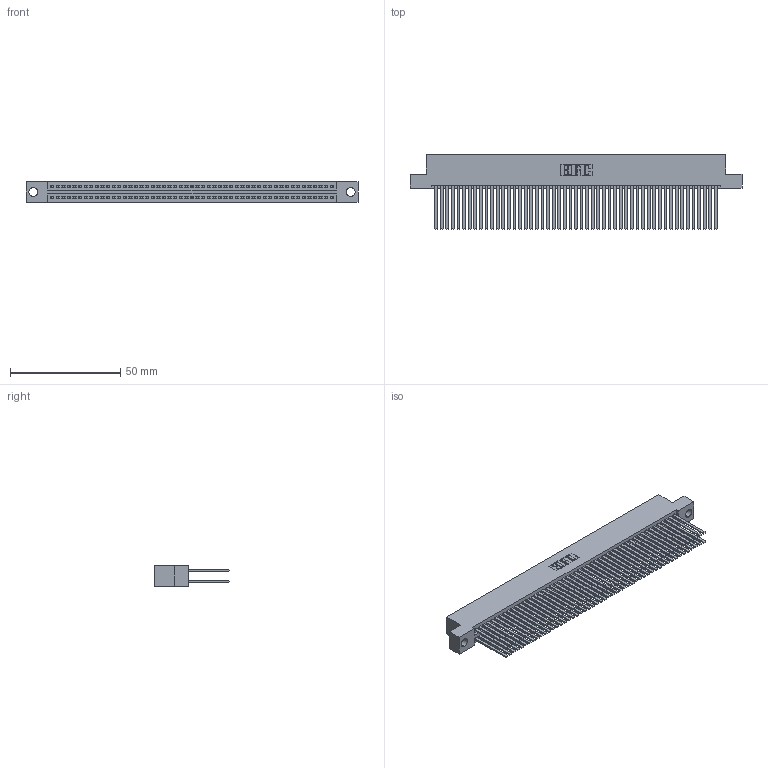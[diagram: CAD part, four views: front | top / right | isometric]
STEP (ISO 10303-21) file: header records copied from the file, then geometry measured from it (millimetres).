
FILE_DESCRIPTION (( 'STEP AP203' ), '1' );
FILE_NAME ('395-102-544-204.STEP', '2018-11-30T08:10:11', ( '' ), ( '' ), 'SwSTEP 2.0', 'SolidWorks 2016', '' );
FILE_SCHEMA (( 'CONFIG_CONTROL_DESIGN' ));
Length unit declared in the file: inch
Products named in the file (3): 345-292-001_345-293-144; 395-102-544-204; 345 Part_Flush Mounting Lugs - 0.156 Dia-TH
Assembly tree (103 placements, depth 2):
  395-102-544-204
    345 Part_Flush Mounting Lugs - 0.156 Dia-TH
    345-292-001_345-293-144  x102
Bounding box: 150.75 x 33.96 x 9.4 mm (x, y, z)
Volume: 16069.4 mm3; surface area: 27933.6 mm2
Topology: 103 solids, 103 shells, 4614 faces, 13703 edges, 8998 vertices
Faces by surface type: plane 3038, cylinder 1576
Entity records: 38623 total; most frequent: CARTESIAN_POINT 6464, ORIENTED_EDGE 6398, DIRECTION 5687, EDGE_CURVE 3199, LINE 2867, VECTOR 2867, VERTEX_POINT 2130, AXIS2_PLACEMENT_3D 1410
